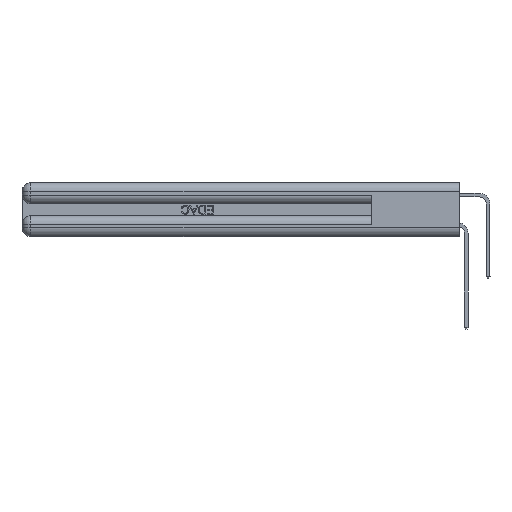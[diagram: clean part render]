
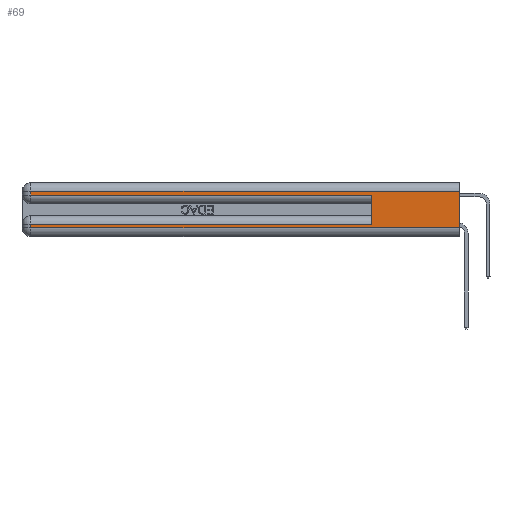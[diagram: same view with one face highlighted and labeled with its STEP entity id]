
A CAD part, left-side view. The second image highlights one B-rep face of the part: STEP entity #69.
In plain terms, the highlighted planar face has unit normal (-1, 0, 0).
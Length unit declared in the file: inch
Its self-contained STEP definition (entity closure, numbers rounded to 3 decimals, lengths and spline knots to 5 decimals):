
#69 = ADVANCED_FACE ( 'NONE', ( #7499 ), #12184, .F. ) ;
#2355 = ORIENTED_EDGE ( 'NONE', *, *, #15567, .T. ) ;
#2388 = CARTESIAN_POINT ( 'NONE',  ( 0., 2.94, 0.37 ) ) ;
#3233 = ORIENTED_EDGE ( 'NONE', *, *, #7796, .T. ) ;
#3848 = ORIENTED_EDGE ( 'NONE', *, *, #39187, .T. ) ;
#4861 = EDGE_CURVE ( 'NONE', #20553, #19015, #44927, .T. ) ;
#5027 = CARTESIAN_POINT ( 'NONE',  ( 0., 0., 0.37 ) ) ;
#5032 = VERTEX_POINT ( 'NONE', #26368 ) ;
#5733 = ORIENTED_EDGE ( 'NONE', *, *, #29684, .T. ) ;
#6443 = DIRECTION ( 'NONE',  ( 0., 0., -1. ) ) ;
#6550 = VERTEX_POINT ( 'NONE', #42026 ) ;
#6575 = VECTOR ( 'NONE', #38202, 39.37008 ) ;
#7499 = FACE_OUTER_BOUND ( 'NONE', #26929, .T. ) ;
#7796 = EDGE_CURVE ( 'NONE', #19015, #26950, #10224, .T. ) ;
#9033 = CARTESIAN_POINT ( 'NONE',  ( 0., 2.94, 0.085 ) ) ;
#10224 = LINE ( 'NONE', #45827, #20724 ) ;
#10494 = CARTESIAN_POINT ( 'NONE',  ( 0., 2.94, 0.285 ) ) ;
#11439 = VECTOR ( 'NONE', #38865, 39.37008 ) ;
#11597 = DIRECTION ( 'NONE',  ( 0., 0., 1. ) ) ;
#12081 = DIRECTION ( 'NONE',  ( 0., -1., 0. ) ) ;
#12184 = PLANE ( 'NONE',  #15521 ) ;
#13787 = ORIENTED_EDGE ( 'NONE', *, *, #4861, .T. ) ;
#14197 = LINE ( 'NONE', #43683, #22921 ) ;
#14419 = CARTESIAN_POINT ( 'NONE',  ( 0., 0., 0.31 ) ) ;
#15095 = CARTESIAN_POINT ( 'NONE',  ( 0., 2.94, 0.06 ) ) ;
#15521 = AXIS2_PLACEMENT_3D ( 'NONE', #5027, #38225, #23434 ) ;
#15567 = EDGE_CURVE ( 'NONE', #27984, #20074, #41161, .T. ) ;
#15778 = CARTESIAN_POINT ( 'NONE',  ( 0., 0., 0.285 ) ) ;
#15950 = DIRECTION ( 'NONE',  ( 0., -1., 0. ) ) ;
#17478 = DIRECTION ( 'NONE',  ( 0., 0., -1. ) ) ;
#17543 = CARTESIAN_POINT ( 'NONE',  ( 0., 2.94, 0.37 ) ) ;
#19015 = VERTEX_POINT ( 'NONE', #15095 ) ;
#19256 = VECTOR ( 'NONE', #15950, 39.37008 ) ;
#20074 = VERTEX_POINT ( 'NONE', #10494 ) ;
#20553 = VERTEX_POINT ( 'NONE', #9033 ) ;
#20724 = VECTOR ( 'NONE', #12081, 39.37008 ) ;
#22921 = VECTOR ( 'NONE', #17478, 39.37008 ) ;
#23434 = DIRECTION ( 'NONE',  ( 0., 0., -1. ) ) ;
#24420 = ORIENTED_EDGE ( 'NONE', *, *, #25355, .F. ) ;
#24994 = CARTESIAN_POINT ( 'NONE',  ( 0., 2.94, 0.31 ) ) ;
#25355 = EDGE_CURVE ( 'NONE', #6550, #26950, #14197, .T. ) ;
#26368 = CARTESIAN_POINT ( 'NONE',  ( 0., 0.6, 0.285 ) ) ;
#26789 = ORIENTED_EDGE ( 'NONE', *, *, #47536, .F. ) ;
#26929 = EDGE_LOOP ( 'NONE', ( #24420, #31274, #2355, #3848, #26789, #5733, #13787, #3233 ) ) ;
#26950 = VERTEX_POINT ( 'NONE', #41068 ) ;
#27984 = VERTEX_POINT ( 'NONE', #24994 ) ;
#29045 = DIRECTION ( 'NONE',  ( 0., 1., 0. ) ) ;
#29684 = EDGE_CURVE ( 'NONE', #33946, #20553, #43319, .T. ) ;
#31274 = ORIENTED_EDGE ( 'NONE', *, *, #47418, .T. ) ;
#33946 = VERTEX_POINT ( 'NONE', #45272 ) ;
#34344 = LINE ( 'NONE', #14419, #44869 ) ;
#36129 = VECTOR ( 'NONE', #6443, 39.37008 ) ;
#38202 = DIRECTION ( 'NONE',  ( 0., 1., 0. ) ) ;
#38225 = DIRECTION ( 'NONE',  ( 1., 0., 0. ) ) ;
#38865 = DIRECTION ( 'NONE',  ( 0., 0., -1. ) ) ;
#39036 = LINE ( 'NONE', #45367, #43128 ) ;
#39187 = EDGE_CURVE ( 'NONE', #20074, #5032, #41912, .T. ) ;
#41068 = CARTESIAN_POINT ( 'NONE',  ( 0., 0., 0.06 ) ) ;
#41161 = LINE ( 'NONE', #2388, #11439 ) ;
#41791 = CARTESIAN_POINT ( 'NONE',  ( 0., 0., 0.085 ) ) ;
#41912 = LINE ( 'NONE', #15778, #19256 ) ;
#42026 = CARTESIAN_POINT ( 'NONE',  ( 0., 0., 0.31 ) ) ;
#43128 = VECTOR ( 'NONE', #11597, 39.37008 ) ;
#43319 = LINE ( 'NONE', #41791, #6575 ) ;
#43683 = CARTESIAN_POINT ( 'NONE',  ( 0., 0., 0.37 ) ) ;
#44869 = VECTOR ( 'NONE', #29045, 39.37008 ) ;
#44927 = LINE ( 'NONE', #17543, #36129 ) ;
#45272 = CARTESIAN_POINT ( 'NONE',  ( 0., 0.6, 0.085 ) ) ;
#45367 = CARTESIAN_POINT ( 'NONE',  ( 0., 0.6, 0.145 ) ) ;
#45827 = CARTESIAN_POINT ( 'NONE',  ( 0., 0., 0.06 ) ) ;
#47418 = EDGE_CURVE ( 'NONE', #6550, #27984, #34344, .T. ) ;
#47536 = EDGE_CURVE ( 'NONE', #33946, #5032, #39036, .T. ) ;
